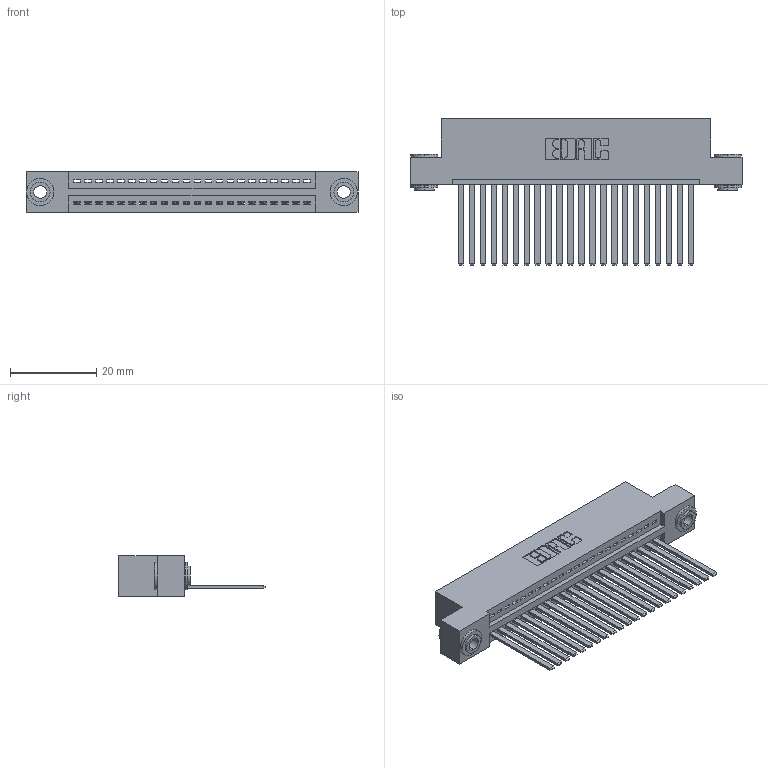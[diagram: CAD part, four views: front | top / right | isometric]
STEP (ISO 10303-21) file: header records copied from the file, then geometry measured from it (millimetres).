
FILE_DESCRIPTION (( 'STEP AP203' ), '1' );
FILE_NAME ('395-022-544-103.STEP', '2019-10-18T03:39:03', ( '' ), ( '' ), 'SwSTEP 2.0', 'SolidWorks 2016', '' );
FILE_SCHEMA (( 'CONFIG_CONTROL_DESIGN' ));
Length unit declared in the file: inch
Products named in the file (4): 345-250-002_345-250-002-102; 345-292-001_345-293-144; 345 Part_Flush Mounting Lugs - 0.156 Dia-TH; 395-022-544-103
Assembly tree (25 placements, depth 2):
  395-022-544-103
    345 Part_Flush Mounting Lugs - 0.156 Dia-TH
    345-292-001_345-293-144  x22
    345-250-002_345-250-002-102  x2
Bounding box: 77.09 x 33.96 x 9.4 mm (x, y, z)
Volume: 7432.3 mm3; surface area: 10584.5 mm2
Topology: 25 solids, 25 shells, 1308 faces, 3893 edges, 2562 vertices
Faces by surface type: plane 882, cylinder 418, cone 8
Entity records: 19716 total; most frequent: CARTESIAN_POINT 3393, ORIENTED_EDGE 3342, DIRECTION 3021, EDGE_CURVE 1671, VECTOR 1431, LINE 1431, VERTEX_POINT 1110, AXIS2_PLACEMENT_3D 795
